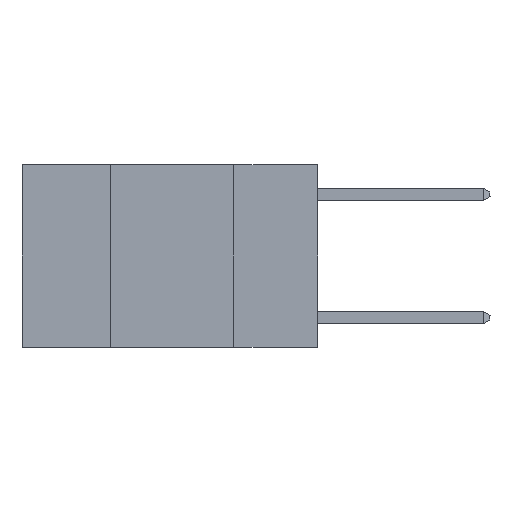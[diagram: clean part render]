
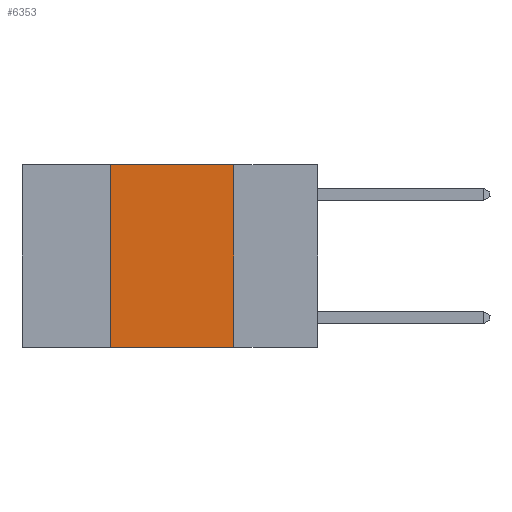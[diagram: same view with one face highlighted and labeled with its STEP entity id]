
A CAD part, left-side view. The second image highlights one B-rep face of the part: STEP entity #6353.
In plain terms, the highlighted planar face has unit normal (-1, 0, 0).
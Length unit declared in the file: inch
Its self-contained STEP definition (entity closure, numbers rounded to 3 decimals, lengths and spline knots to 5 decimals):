
#353 = CARTESIAN_POINT ( 'NONE',  ( 0., 0.6, 0. ) ) ;
#772 = EDGE_CURVE ( 'NONE', #8861, #4997, #1641, .T. ) ;
#995 = LINE ( 'NONE', #3809, #2956 ) ;
#1138 = CARTESIAN_POINT ( 'NONE',  ( 0., 0.42, 0. ) ) ;
#1333 = DIRECTION ( 'NONE',  ( 1., 0., 0. ) ) ;
#1603 = CARTESIAN_POINT ( 'NONE',  ( 0., 0.42, -0.37 ) ) ;
#1641 = LINE ( 'NONE', #9806, #9398 ) ;
#1805 = EDGE_CURVE ( 'NONE', #4997, #9319, #995, .T. ) ;
#2010 = ORIENTED_EDGE ( 'NONE', *, *, #12406, .F. ) ;
#2956 = VECTOR ( 'NONE', #10648, 39.37008 ) ;
#3809 = CARTESIAN_POINT ( 'NONE',  ( 0., 0.6, 0. ) ) ;
#3986 = VECTOR ( 'NONE', #9388, 39.37008 ) ;
#4891 = ORIENTED_EDGE ( 'NONE', *, *, #772, .F. ) ;
#4997 = VERTEX_POINT ( 'NONE', #1138 ) ;
#6179 = PLANE ( 'NONE',  #10942 ) ;
#6353 = ADVANCED_FACE ( 'NONE', ( #9143 ), #6179, .F. ) ;
#6982 = DIRECTION ( 'NONE',  ( 0., -1., 0. ) ) ;
#7209 = ORIENTED_EDGE ( 'NONE', *, *, #1805, .F. ) ;
#7509 = ORIENTED_EDGE ( 'NONE', *, *, #10777, .T. ) ;
#8139 = DIRECTION ( 'NONE',  ( 0., 0., -1. ) ) ;
#8456 = EDGE_LOOP ( 'NONE', ( #2010, #7209, #4891, #7509 ) ) ;
#8861 = VERTEX_POINT ( 'NONE', #1603 ) ;
#9143 = FACE_OUTER_BOUND ( 'NONE', #8456, .T. ) ;
#9210 = LINE ( 'NONE', #10363, #3986 ) ;
#9319 = VERTEX_POINT ( 'NONE', #11898 ) ;
#9388 = DIRECTION ( 'NONE',  ( 0., 0., -1. ) ) ;
#9398 = VECTOR ( 'NONE', #9596, 39.37008 ) ;
#9596 = DIRECTION ( 'NONE',  ( 0., 0., 1. ) ) ;
#9674 = VECTOR ( 'NONE', #6982, 39.37008 ) ;
#9806 = CARTESIAN_POINT ( 'NONE',  ( 0., 0.42, 0. ) ) ;
#9848 = CARTESIAN_POINT ( 'NONE',  ( 0., 0.6, -0.37 ) ) ;
#10363 = CARTESIAN_POINT ( 'NONE',  ( 0., 0.17, 0. ) ) ;
#10499 = VERTEX_POINT ( 'NONE', #10785 ) ;
#10648 = DIRECTION ( 'NONE',  ( 0., -1., 0. ) ) ;
#10777 = EDGE_CURVE ( 'NONE', #8861, #10499, #12242, .T. ) ;
#10785 = CARTESIAN_POINT ( 'NONE',  ( 0., 0.17, -0.37 ) ) ;
#10942 = AXIS2_PLACEMENT_3D ( 'NONE', #353, #1333, #8139 ) ;
#11898 = CARTESIAN_POINT ( 'NONE',  ( 0., 0.17, 0. ) ) ;
#12242 = LINE ( 'NONE', #9848, #9674 ) ;
#12406 = EDGE_CURVE ( 'NONE', #9319, #10499, #9210, .T. ) ;
